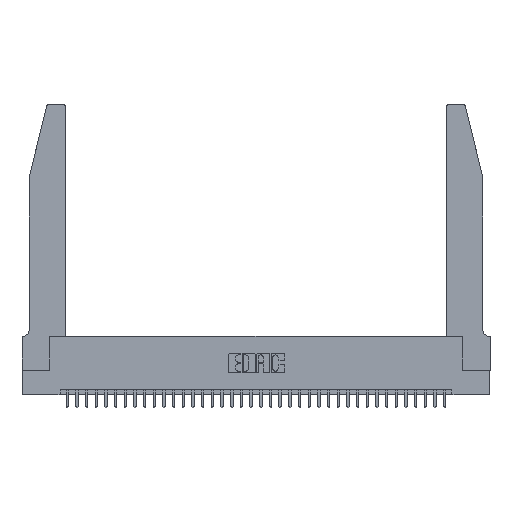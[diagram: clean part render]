
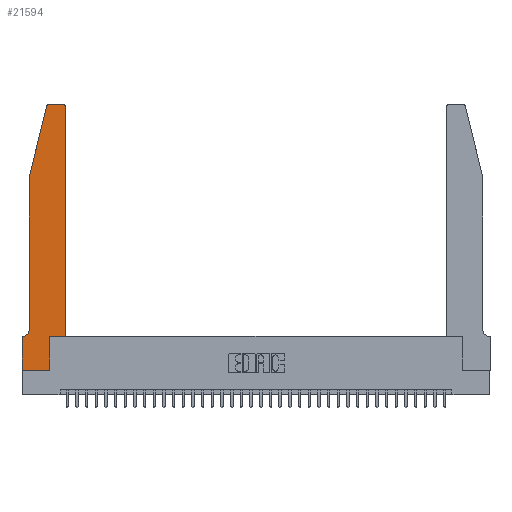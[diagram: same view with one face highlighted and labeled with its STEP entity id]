
A CAD part, top view. The second image highlights one B-rep face of the part: STEP entity #21594.
In plain terms, the highlighted planar face has unit normal (0, 0, 1).
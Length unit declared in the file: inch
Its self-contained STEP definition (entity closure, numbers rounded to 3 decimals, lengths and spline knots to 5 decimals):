
#5 = CARTESIAN_POINT ( 'NONE',  ( 0.4205, 2.75, 0.37 ) ) ;
#141 = VECTOR ( 'NONE', #22025, 39.37008 ) ;
#265 = CIRCLE ( 'NONE', #33333, 0.07 ) ;
#745 = CARTESIAN_POINT ( 'NONE',  ( 0., 0., 0.37 ) ) ;
#839 = LINE ( 'NONE', #22468, #14994 ) ;
#863 = DIRECTION ( 'NONE',  ( -1., 0., 0. ) ) ;
#2033 = ORIENTED_EDGE ( 'NONE', *, *, #3909, .T. ) ;
#3059 = CARTESIAN_POINT ( 'NONE',  ( 0.4505, 2.72, 0.37 ) ) ;
#3152 = VERTEX_POINT ( 'NONE', #15850 ) ;
#3232 = CARTESIAN_POINT ( 'NONE',  ( 0., 0., 0.37 ) ) ;
#3496 = VERTEX_POINT ( 'NONE', #33980 ) ;
#3658 = EDGE_CURVE ( 'NONE', #25578, #3496, #11245, .T. ) ;
#3805 = ORIENTED_EDGE ( 'NONE', *, *, #13723, .T. ) ;
#3909 = EDGE_CURVE ( 'NONE', #19989, #3152, #16503, .T. ) ;
#4077 = CARTESIAN_POINT ( 'NONE',  ( 0.0055, 0.42, 0.37 ) ) ;
#5780 = AXIS2_PLACEMENT_3D ( 'NONE', #11477, #31092, #14320 ) ;
#5855 = VERTEX_POINT ( 'NONE', #13604 ) ;
#6074 = EDGE_CURVE ( 'NONE', #5855, #25578, #265, .T. ) ;
#6724 = LINE ( 'NONE', #15561, #12458 ) ;
#6917 = DIRECTION ( 'NONE',  ( -1., 0., 0. ) ) ;
#6965 = LINE ( 'NONE', #8152, #28489 ) ;
#8152 = CARTESIAN_POINT ( 'NONE',  ( 0.0755, 2., 0.37 ) ) ;
#8193 = CARTESIAN_POINT ( 'NONE',  ( 0.4505, 0.35, 0.37 ) ) ;
#8977 = ORIENTED_EDGE ( 'NONE', *, *, #36021, .T. ) ;
#9377 = CIRCLE ( 'NONE', #22595, 0.03 ) ;
#10134 = ORIENTED_EDGE ( 'NONE', *, *, #3658, .T. ) ;
#10373 = CARTESIAN_POINT ( 'NONE',  ( 0.25487, 2.72718, 0.37 ) ) ;
#10728 = AXIS2_PLACEMENT_3D ( 'NONE', #16716, #36355, #19540 ) ;
#10790 = ORIENTED_EDGE ( 'NONE', *, *, #30776, .T. ) ;
#11245 = LINE ( 'NONE', #34689, #32737 ) ;
#11361 = PLANE ( 'NONE',  #5780 ) ;
#11477 = CARTESIAN_POINT ( 'NONE',  ( 0., 0.35, 0.37 ) ) ;
#11514 = CARTESIAN_POINT ( 'NONE',  ( 0.2865, 0., 0.37 ) ) ;
#11897 = EDGE_LOOP ( 'NONE', ( #8977, #21175, #10790, #12304, #22149, #10134, #33435, #20636, #2033, #32807, #27206, #3805 ) ) ;
#12236 = DIRECTION ( 'NONE',  ( 1., 0., 0. ) ) ;
#12304 = ORIENTED_EDGE ( 'NONE', *, *, #21203, .T. ) ;
#12314 = EDGE_CURVE ( 'NONE', #35630, #18810, #30088, .T. ) ;
#12458 = VECTOR ( 'NONE', #18362, 39.37008 ) ;
#13480 = DIRECTION ( 'NONE',  ( 0., 1., 0. ) ) ;
#13604 = CARTESIAN_POINT ( 'NONE',  ( 0.0755, 0.42, 0.37 ) ) ;
#13723 = EDGE_CURVE ( 'NONE', #18810, #22842, #9377, .T. ) ;
#14098 = DIRECTION ( 'NONE',  ( 0., 0., 1. ) ) ;
#14320 = DIRECTION ( 'NONE',  ( 1., 0., 0. ) ) ;
#14994 = VECTOR ( 'NONE', #17061, 39.37008 ) ;
#15059 = FACE_OUTER_BOUND ( 'NONE', #11897, .T. ) ;
#15561 = CARTESIAN_POINT ( 'NONE',  ( 0.0755, 2., 0.37 ) ) ;
#15850 = CARTESIAN_POINT ( 'NONE',  ( 0.2865, 0.35, 0.37 ) ) ;
#16334 = DIRECTION ( 'NONE',  ( 0., -1., 0. ) ) ;
#16503 = LINE ( 'NONE', #30258, #17373 ) ;
#16716 = CARTESIAN_POINT ( 'NONE',  ( 0.284, 2.72, 0.37 ) ) ;
#17061 = DIRECTION ( 'NONE',  ( -1., 0., 0. ) ) ;
#17373 = VECTOR ( 'NONE', #13480, 39.37008 ) ;
#18362 = DIRECTION ( 'NONE',  ( 0., -1., 0. ) ) ;
#18535 = VERTEX_POINT ( 'NONE', #10373 ) ;
#18810 = VERTEX_POINT ( 'NONE', #3059 ) ;
#19230 = EDGE_CURVE ( 'NONE', #29726, #18535, #26205, .T. ) ;
#19273 = LINE ( 'NONE', #26210, #32404 ) ;
#19540 = DIRECTION ( 'NONE',  ( 1., 0., 0. ) ) ;
#19989 = VERTEX_POINT ( 'NONE', #11514 ) ;
#20031 = VERTEX_POINT ( 'NONE', #3232 ) ;
#20636 = ORIENTED_EDGE ( 'NONE', *, *, #36217, .T. ) ;
#20753 = CARTESIAN_POINT ( 'NONE',  ( 0.4505, 0.35, 0.37 ) ) ;
#20810 = CARTESIAN_POINT ( 'NONE',  ( 0.284, 2.75, 0.37 ) ) ;
#21175 = ORIENTED_EDGE ( 'NONE', *, *, #19230, .T. ) ;
#21203 = EDGE_CURVE ( 'NONE', #35309, #5855, #6724, .T. ) ;
#21594 = ADVANCED_FACE ( 'NONE', ( #15059 ), #11361, .T. ) ;
#22025 = DIRECTION ( 'NONE',  ( 0., 1., 0. ) ) ;
#22111 = CARTESIAN_POINT ( 'NONE',  ( 0.0755, 2., 0.37 ) ) ;
#22149 = ORIENTED_EDGE ( 'NONE', *, *, #6074, .T. ) ;
#22468 = CARTESIAN_POINT ( 'NONE',  ( 0.2605, 2.75, 0.37 ) ) ;
#22595 = AXIS2_PLACEMENT_3D ( 'NONE', #30882, #14098, #33718 ) ;
#22842 = VERTEX_POINT ( 'NONE', #5 ) ;
#23731 = DIRECTION ( 'NONE',  ( 0., 0., -1. ) ) ;
#24643 = VECTOR ( 'NONE', #28922, 39.37008 ) ;
#24664 = CARTESIAN_POINT ( 'NONE',  ( 0., 0., 0.37 ) ) ;
#24925 = DIRECTION ( 'NONE',  ( -0.239, -0.971, 0. ) ) ;
#25578 = VERTEX_POINT ( 'NONE', #27460 ) ;
#26205 = CIRCLE ( 'NONE', #10728, 0.03 ) ;
#26210 = CARTESIAN_POINT ( 'NONE',  ( 0.4505, 0.35, 0.37 ) ) ;
#27206 = ORIENTED_EDGE ( 'NONE', *, *, #12314, .T. ) ;
#27460 = CARTESIAN_POINT ( 'NONE',  ( 0.0055, 0.35, 0.37 ) ) ;
#28459 = VECTOR ( 'NONE', #16334, 39.37008 ) ;
#28489 = VECTOR ( 'NONE', #24925, 39.37008 ) ;
#28922 = DIRECTION ( 'NONE',  ( 1., 0., 0. ) ) ;
#29690 = EDGE_CURVE ( 'NONE', #3152, #35630, #19273, .T. ) ;
#29726 = VERTEX_POINT ( 'NONE', #20810 ) ;
#30088 = LINE ( 'NONE', #8193, #141 ) ;
#30258 = CARTESIAN_POINT ( 'NONE',  ( 0.2865, 0.35, 0.37 ) ) ;
#30776 = EDGE_CURVE ( 'NONE', #18535, #35309, #6965, .T. ) ;
#30882 = CARTESIAN_POINT ( 'NONE',  ( 0.4205, 2.72, 0.37 ) ) ;
#31092 = DIRECTION ( 'NONE',  ( 0., 0., 1. ) ) ;
#31249 = EDGE_CURVE ( 'NONE', #3496, #20031, #35034, .T. ) ;
#32065 = LINE ( 'NONE', #745, #24643 ) ;
#32404 = VECTOR ( 'NONE', #12236, 39.37008 ) ;
#32737 = VECTOR ( 'NONE', #863, 39.37008 ) ;
#32807 = ORIENTED_EDGE ( 'NONE', *, *, #29690, .T. ) ;
#33333 = AXIS2_PLACEMENT_3D ( 'NONE', #4077, #23731, #6917 ) ;
#33435 = ORIENTED_EDGE ( 'NONE', *, *, #31249, .T. ) ;
#33718 = DIRECTION ( 'NONE',  ( 1., 0., 0. ) ) ;
#33980 = CARTESIAN_POINT ( 'NONE',  ( 0., 0.35, 0.37 ) ) ;
#34689 = CARTESIAN_POINT ( 'NONE',  ( 0.0755, 0.35, 0.37 ) ) ;
#35034 = LINE ( 'NONE', #24664, #28459 ) ;
#35309 = VERTEX_POINT ( 'NONE', #22111 ) ;
#35630 = VERTEX_POINT ( 'NONE', #20753 ) ;
#36021 = EDGE_CURVE ( 'NONE', #22842, #29726, #839, .T. ) ;
#36217 = EDGE_CURVE ( 'NONE', #20031, #19989, #32065, .T. ) ;
#36355 = DIRECTION ( 'NONE',  ( 0., 0., 1. ) ) ;
